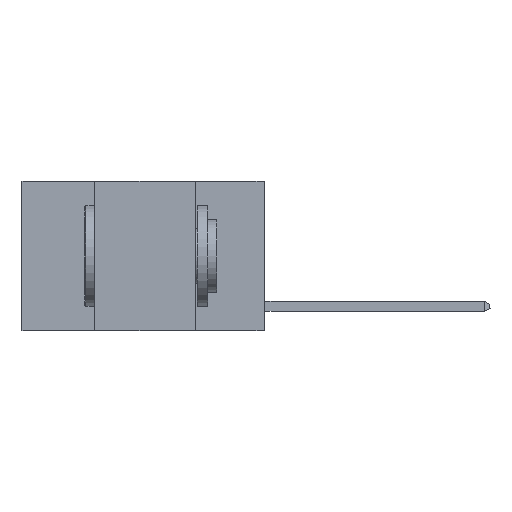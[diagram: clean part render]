
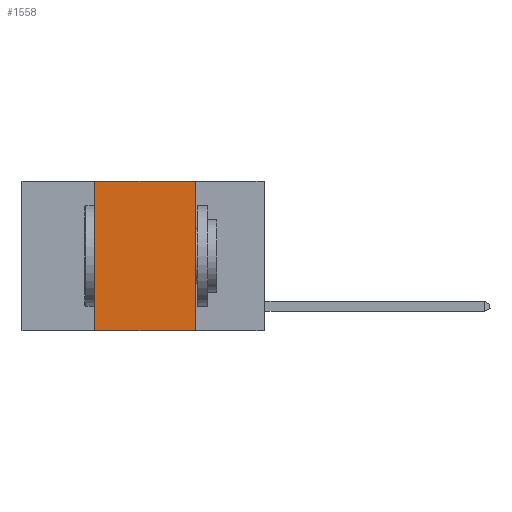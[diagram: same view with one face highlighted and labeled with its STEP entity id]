
A CAD part, left-side view. The second image highlights one B-rep face of the part: STEP entity #1558.
In plain terms, the highlighted planar face has unit normal (-1, 0, 0).
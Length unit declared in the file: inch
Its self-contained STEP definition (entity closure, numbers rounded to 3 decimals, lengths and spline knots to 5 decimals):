
#310 = EDGE_CURVE ( 'NONE', #18151, #9717, #13785, .T. ) ;
#611 = CARTESIAN_POINT ( 'NONE',  ( 0., 0.6, 0. ) ) ;
#628 = VECTOR ( 'NONE', #2547, 39.37008 ) ;
#824 = VERTEX_POINT ( 'NONE', #6593 ) ;
#1363 = EDGE_LOOP ( 'NONE', ( #8256, #12556, #13696, #7941 ) ) ;
#1558 = ADVANCED_FACE ( 'NONE', ( #20912 ), #3516, .F. ) ;
#2421 = CARTESIAN_POINT ( 'NONE',  ( 0., 0.6, -0.37 ) ) ;
#2547 = DIRECTION ( 'NONE',  ( 0., -1., 0. ) ) ;
#3516 = PLANE ( 'NONE',  #6662 ) ;
#3889 = DIRECTION ( 'NONE',  ( 0., 0., -1. ) ) ;
#4840 = VECTOR ( 'NONE', #10196, 39.37008 ) ;
#6593 = CARTESIAN_POINT ( 'NONE',  ( 0., 0.17, 0. ) ) ;
#6662 = AXIS2_PLACEMENT_3D ( 'NONE', #22676, #18912, #22798 ) ;
#6754 = EDGE_CURVE ( 'NONE', #18151, #9188, #7215, .T. ) ;
#7010 = EDGE_CURVE ( 'NONE', #9188, #824, #23544, .T. ) ;
#7215 = LINE ( 'NONE', #12841, #18921 ) ;
#7572 = LINE ( 'NONE', #24876, #10037 ) ;
#7941 = ORIENTED_EDGE ( 'NONE', *, *, #310, .T. ) ;
#8256 = ORIENTED_EDGE ( 'NONE', *, *, #19720, .F. ) ;
#9188 = VERTEX_POINT ( 'NONE', #16503 ) ;
#9717 = VERTEX_POINT ( 'NONE', #22125 ) ;
#10037 = VECTOR ( 'NONE', #3889, 39.37008 ) ;
#10196 = DIRECTION ( 'NONE',  ( 0., -1., 0. ) ) ;
#10817 = DIRECTION ( 'NONE',  ( 0., 0., 1. ) ) ;
#12556 = ORIENTED_EDGE ( 'NONE', *, *, #7010, .F. ) ;
#12841 = CARTESIAN_POINT ( 'NONE',  ( 0., 0.42, 0. ) ) ;
#13696 = ORIENTED_EDGE ( 'NONE', *, *, #6754, .F. ) ;
#13785 = LINE ( 'NONE', #2421, #628 ) ;
#16503 = CARTESIAN_POINT ( 'NONE',  ( 0., 0.42, 0. ) ) ;
#18026 = CARTESIAN_POINT ( 'NONE',  ( 0., 0.42, -0.37 ) ) ;
#18151 = VERTEX_POINT ( 'NONE', #18026 ) ;
#18912 = DIRECTION ( 'NONE',  ( 1., 0., 0. ) ) ;
#18921 = VECTOR ( 'NONE', #10817, 39.37008 ) ;
#19720 = EDGE_CURVE ( 'NONE', #824, #9717, #7572, .T. ) ;
#20912 = FACE_OUTER_BOUND ( 'NONE', #1363, .T. ) ;
#22125 = CARTESIAN_POINT ( 'NONE',  ( 0., 0.17, -0.37 ) ) ;
#22676 = CARTESIAN_POINT ( 'NONE',  ( 0., 0.6, 0. ) ) ;
#22798 = DIRECTION ( 'NONE',  ( 0., 0., -1. ) ) ;
#23544 = LINE ( 'NONE', #611, #4840 ) ;
#24876 = CARTESIAN_POINT ( 'NONE',  ( 0., 0.17, 0. ) ) ;
